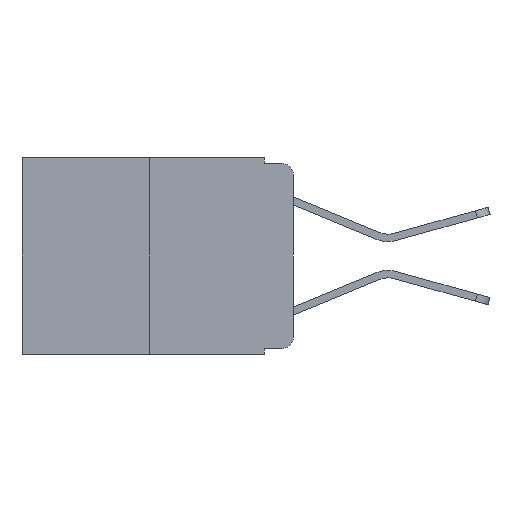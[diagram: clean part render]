
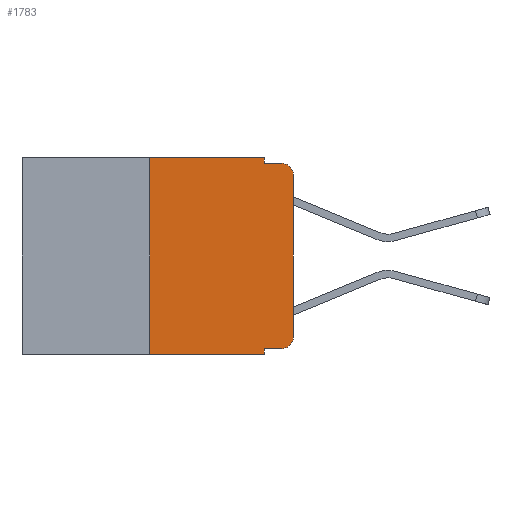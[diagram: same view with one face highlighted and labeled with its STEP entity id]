
A CAD part, left-side view. The second image highlights one B-rep face of the part: STEP entity #1783.
In plain terms, the highlighted planar face has unit normal (-1, 0, 0).
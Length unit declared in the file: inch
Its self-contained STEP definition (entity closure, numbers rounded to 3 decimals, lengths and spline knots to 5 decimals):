
#38 = AXIS2_PLACEMENT_3D ( 'NONE', #10906, #9529, #1177 ) ;
#354 = ORIENTED_EDGE ( 'NONE', *, *, #8769, .T. ) ;
#431 = CARTESIAN_POINT ( 'NONE',  ( 0., 0.051, 0. ) ) ;
#449 = DIRECTION ( 'NONE',  ( 0., -1., 0. ) ) ;
#562 = LINE ( 'NONE', #985, #8688 ) ;
#985 = CARTESIAN_POINT ( 'NONE',  ( 0., 0.25, 0. ) ) ;
#995 = VERTEX_POINT ( 'NONE', #1803 ) ;
#1177 = DIRECTION ( 'NONE',  ( 0., 0., -1. ) ) ;
#1783 = ADVANCED_FACE ( 'NONE', ( #4090 ), #11015, .F. ) ;
#1803 = CARTESIAN_POINT ( 'NONE',  ( 0., 0., -0.313 ) ) ;
#2226 = AXIS2_PLACEMENT_3D ( 'NONE', #4500, #10958, #5569 ) ;
#2269 = CARTESIAN_POINT ( 'NONE',  ( 0., 0.051, -0.333 ) ) ;
#2300 = CARTESIAN_POINT ( 'NONE',  ( 0., 0.473, 0. ) ) ;
#2345 = VERTEX_POINT ( 'NONE', #2689 ) ;
#2689 = CARTESIAN_POINT ( 'NONE',  ( 0., 0., -0.03 ) ) ;
#2710 = CARTESIAN_POINT ( 'NONE',  ( 0., 0.051, -0.343 ) ) ;
#2744 = VERTEX_POINT ( 'NONE', #9192 ) ;
#3129 = VERTEX_POINT ( 'NONE', #12348 ) ;
#3186 = ORIENTED_EDGE ( 'NONE', *, *, #4975, .T. ) ;
#3324 = ORIENTED_EDGE ( 'NONE', *, *, #7380, .F. ) ;
#3432 = VERTEX_POINT ( 'NONE', #6007 ) ;
#3451 = CARTESIAN_POINT ( 'NONE',  ( 0., 0.051, -0.333 ) ) ;
#3495 = VECTOR ( 'NONE', #449, 39.37008 ) ;
#3528 = ORIENTED_EDGE ( 'NONE', *, *, #9669, .F. ) ;
#3573 = VECTOR ( 'NONE', #10321, 39.37008 ) ;
#3612 = CARTESIAN_POINT ( 'NONE',  ( 0., 0.051, 0. ) ) ;
#3701 = CARTESIAN_POINT ( 'NONE',  ( 0., 0.051, -0.01 ) ) ;
#3838 = ORIENTED_EDGE ( 'NONE', *, *, #5860, .F. ) ;
#3850 = AXIS2_PLACEMENT_3D ( 'NONE', #10943, #5546, #11787 ) ;
#3866 = LINE ( 'NONE', #12043, #3495 ) ;
#4032 = LINE ( 'NONE', #3612, #9122 ) ;
#4090 = FACE_OUTER_BOUND ( 'NONE', #5208, .T. ) ;
#4406 = LINE ( 'NONE', #9772, #6762 ) ;
#4464 = VERTEX_POINT ( 'NONE', #9890 ) ;
#4500 = CARTESIAN_POINT ( 'NONE',  ( 0., 0.02, -0.313 ) ) ;
#4703 = ORIENTED_EDGE ( 'NONE', *, *, #8984, .T. ) ;
#4975 = EDGE_CURVE ( 'NONE', #3432, #995, #7056, .T. ) ;
#5208 = EDGE_LOOP ( 'NONE', ( #354, #4703, #3324, #3528, #12005, #3838, #10471, #11077, #6845, #3186 ) ) ;
#5546 = DIRECTION ( 'NONE',  ( -1., 0., 0. ) ) ;
#5569 = DIRECTION ( 'NONE',  ( 0., 0., -1. ) ) ;
#5860 = EDGE_CURVE ( 'NONE', #3129, #2744, #562, .T. ) ;
#5939 = EDGE_CURVE ( 'NONE', #2744, #9987, #11934, .T. ) ;
#6007 = CARTESIAN_POINT ( 'NONE',  ( 0., 0.02, -0.333 ) ) ;
#6013 = CARTESIAN_POINT ( 'NONE',  ( 0., 0.051, -0.01 ) ) ;
#6109 = EDGE_CURVE ( 'NONE', #12458, #9411, #4032, .T. ) ;
#6294 = CARTESIAN_POINT ( 'NONE',  ( 0., 0., 0. ) ) ;
#6337 = DIRECTION ( 'NONE',  ( 0., 0., 1. ) ) ;
#6564 = DIRECTION ( 'NONE',  ( 0., -1., 0. ) ) ;
#6644 = LINE ( 'NONE', #3701, #3573 ) ;
#6762 = VECTOR ( 'NONE', #7106, 39.37008 ) ;
#6845 = ORIENTED_EDGE ( 'NONE', *, *, #8236, .T. ) ;
#7056 = CIRCLE ( 'NONE', #2226, 0.02 ) ;
#7106 = DIRECTION ( 'NONE',  ( 0., 0., -1. ) ) ;
#7380 = EDGE_CURVE ( 'NONE', #10181, #4464, #6644, .T. ) ;
#7743 = CIRCLE ( 'NONE', #3850, 0.02 ) ;
#8236 = EDGE_CURVE ( 'NONE', #12458, #3432, #11848, .T. ) ;
#8584 = VECTOR ( 'NONE', #9900, 39.37008 ) ;
#8688 = VECTOR ( 'NONE', #6337, 39.37008 ) ;
#8769 = EDGE_CURVE ( 'NONE', #995, #2345, #10925, .T. ) ;
#8984 = EDGE_CURVE ( 'NONE', #2345, #4464, #7743, .T. ) ;
#9122 = VECTOR ( 'NONE', #11958, 39.37008 ) ;
#9192 = CARTESIAN_POINT ( 'NONE',  ( 0., 0.25, 0. ) ) ;
#9411 = VERTEX_POINT ( 'NONE', #2710 ) ;
#9529 = DIRECTION ( 'NONE',  ( 1., 0., 0. ) ) ;
#9589 = VECTOR ( 'NONE', #10952, 39.37008 ) ;
#9669 = EDGE_CURVE ( 'NONE', #9987, #10181, #4406, .T. ) ;
#9682 = VECTOR ( 'NONE', #6564, 39.37008 ) ;
#9772 = CARTESIAN_POINT ( 'NONE',  ( 0., 0.051, 0. ) ) ;
#9890 = CARTESIAN_POINT ( 'NONE',  ( 0., 0.02, -0.01 ) ) ;
#9900 = DIRECTION ( 'NONE',  ( 0., 0., 1. ) ) ;
#9987 = VERTEX_POINT ( 'NONE', #431 ) ;
#10181 = VERTEX_POINT ( 'NONE', #6013 ) ;
#10321 = DIRECTION ( 'NONE',  ( 0., -1., 0. ) ) ;
#10471 = ORIENTED_EDGE ( 'NONE', *, *, #12041, .T. ) ;
#10906 = CARTESIAN_POINT ( 'NONE',  ( 0., 0.473, 0. ) ) ;
#10925 = LINE ( 'NONE', #6294, #8584 ) ;
#10943 = CARTESIAN_POINT ( 'NONE',  ( 0., 0.02, -0.03 ) ) ;
#10952 = DIRECTION ( 'NONE',  ( 0., -1., 0. ) ) ;
#10958 = DIRECTION ( 'NONE',  ( -1., 0., 0. ) ) ;
#11015 = PLANE ( 'NONE',  #38 ) ;
#11077 = ORIENTED_EDGE ( 'NONE', *, *, #6109, .F. ) ;
#11787 = DIRECTION ( 'NONE',  ( 0., 0., -1. ) ) ;
#11848 = LINE ( 'NONE', #2269, #9589 ) ;
#11934 = LINE ( 'NONE', #2300, #9682 ) ;
#11958 = DIRECTION ( 'NONE',  ( 0., 0., -1. ) ) ;
#12005 = ORIENTED_EDGE ( 'NONE', *, *, #5939, .F. ) ;
#12041 = EDGE_CURVE ( 'NONE', #3129, #9411, #3866, .T. ) ;
#12043 = CARTESIAN_POINT ( 'NONE',  ( 0., 0.473, -0.343 ) ) ;
#12348 = CARTESIAN_POINT ( 'NONE',  ( 0., 0.25, -0.343 ) ) ;
#12458 = VERTEX_POINT ( 'NONE', #3451 ) ;
